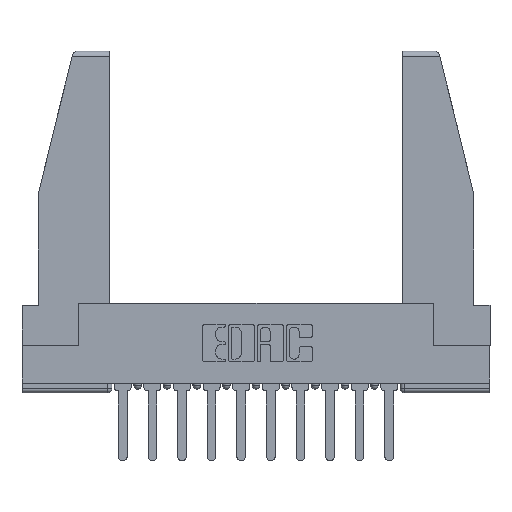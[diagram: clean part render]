
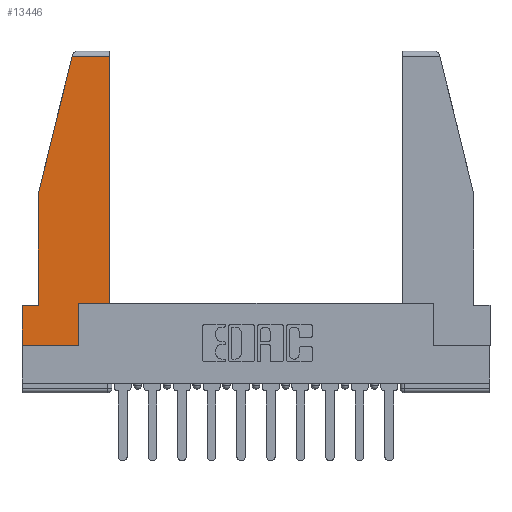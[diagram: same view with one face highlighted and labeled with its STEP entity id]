
A CAD part, top view. The second image highlights one B-rep face of the part: STEP entity #13446.
In plain terms, the highlighted planar face has unit normal (0, 0, 1).
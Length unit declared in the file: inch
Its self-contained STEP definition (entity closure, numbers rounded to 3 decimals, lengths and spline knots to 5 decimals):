
#3 = AXIS2_PLACEMENT_3D ( 'NONE', #6323, #5048, #13193 ) ;
#172 = VECTOR ( 'NONE', #13600, 39.37008 ) ;
#475 = CARTESIAN_POINT ( 'NONE',  ( 0.086, 0.21, 0. ) ) ;
#1074 = VERTEX_POINT ( 'NONE', #9072 ) ;
#1445 = EDGE_CURVE ( 'NONE', #6165, #9530, #11631, .T. ) ;
#3361 = LINE ( 'NONE', #7458, #3905 ) ;
#3769 = ORIENTED_EDGE ( 'NONE', *, *, #1445, .T. ) ;
#3905 = VECTOR ( 'NONE', #4158, 39.37008 ) ;
#3922 = ORIENTED_EDGE ( 'NONE', *, *, #5482, .T. ) ;
#4035 = VERTEX_POINT ( 'NONE', #12150 ) ;
#4087 = LINE ( 'NONE', #4543, #6825 ) ;
#4092 = VECTOR ( 'NONE', #11732, 39.37008 ) ;
#4114 = EDGE_CURVE ( 'NONE', #6142, #10404, #13201, .T. ) ;
#4158 = DIRECTION ( 'NONE',  ( 0., -1., 0. ) ) ;
#4191 = VERTEX_POINT ( 'NONE', #13590 ) ;
#4446 = EDGE_CURVE ( 'NONE', #4035, #11230, #10036, .T. ) ;
#4543 = CARTESIAN_POINT ( 'NONE',  ( 0.297, 0.223, 0. ) ) ;
#4575 = CARTESIAN_POINT ( 'NONE',  ( 0., 1.52, 0. ) ) ;
#5048 = DIRECTION ( 'NONE',  ( 0., 0., 1. ) ) ;
#5482 = EDGE_CURVE ( 'NONE', #1074, #4035, #9086, .T. ) ;
#5774 = CARTESIAN_POINT ( 'NONE',  ( 0.2636, 1.52, 0. ) ) ;
#5826 = ORIENTED_EDGE ( 'NONE', *, *, #15077, .T. ) ;
#5844 = DIRECTION ( 'NONE',  ( -1., 0., 0. ) ) ;
#5978 = EDGE_CURVE ( 'NONE', #11230, #6165, #7572, .T. ) ;
#6142 = VERTEX_POINT ( 'NONE', #8155 ) ;
#6165 = VERTEX_POINT ( 'NONE', #11639 ) ;
#6323 = CARTESIAN_POINT ( 'NONE',  ( 0., 0., 0. ) ) ;
#6807 = LINE ( 'NONE', #6969, #7715 ) ;
#6825 = VECTOR ( 'NONE', #15157, 39.37008 ) ;
#6947 = CARTESIAN_POINT ( 'NONE',  ( 0.086, 0.8, 0. ) ) ;
#6969 = CARTESIAN_POINT ( 'NONE',  ( 0., 0.21, 0. ) ) ;
#7458 = CARTESIAN_POINT ( 'NONE',  ( 0., 0.21, 0. ) ) ;
#7572 = LINE ( 'NONE', #11406, #14068 ) ;
#7689 = CARTESIAN_POINT ( 'NONE',  ( 0., 0., 0. ) ) ;
#7715 = VECTOR ( 'NONE', #15218, 39.37008 ) ;
#8110 = EDGE_LOOP ( 'NONE', ( #3922, #12747, #13913, #3769, #10765, #10985, #11314, #11056, #5826 ) ) ;
#8155 = CARTESIAN_POINT ( 'NONE',  ( 0., 0., 0. ) ) ;
#8229 = EDGE_CURVE ( 'NONE', #9530, #13166, #6807, .T. ) ;
#8375 = EDGE_CURVE ( 'NONE', #10404, #4191, #12878, .T. ) ;
#8838 = DIRECTION ( 'NONE',  ( 1., 0., 0. ) ) ;
#9072 = CARTESIAN_POINT ( 'NONE',  ( 0.461, 0.223, 0. ) ) ;
#9086 = LINE ( 'NONE', #12764, #11678 ) ;
#9530 = VERTEX_POINT ( 'NONE', #475 ) ;
#10036 = LINE ( 'NONE', #4575, #12995 ) ;
#10243 = DIRECTION ( 'NONE',  ( 0., 1., 0. ) ) ;
#10384 = FACE_OUTER_BOUND ( 'NONE', #8110, .T. ) ;
#10404 = VERTEX_POINT ( 'NONE', #14781 ) ;
#10765 = ORIENTED_EDGE ( 'NONE', *, *, #8229, .T. ) ;
#10985 = ORIENTED_EDGE ( 'NONE', *, *, #14771, .T. ) ;
#11056 = ORIENTED_EDGE ( 'NONE', *, *, #8375, .T. ) ;
#11230 = VERTEX_POINT ( 'NONE', #5774 ) ;
#11314 = ORIENTED_EDGE ( 'NONE', *, *, #4114, .T. ) ;
#11406 = CARTESIAN_POINT ( 'NONE',  ( 0.271, 1.55, 0. ) ) ;
#11545 = VECTOR ( 'NONE', #8838, 39.37008 ) ;
#11631 = LINE ( 'NONE', #6947, #4092 ) ;
#11639 = CARTESIAN_POINT ( 'NONE',  ( 0.086, 0.8, 0. ) ) ;
#11678 = VECTOR ( 'NONE', #10243, 39.37008 ) ;
#11732 = DIRECTION ( 'NONE',  ( 0., -1., 0. ) ) ;
#12103 = PLANE ( 'NONE',  #3 ) ;
#12150 = CARTESIAN_POINT ( 'NONE',  ( 0.461, 1.52, 0. ) ) ;
#12481 = DIRECTION ( 'NONE',  ( -0.239, -0.971, 0. ) ) ;
#12747 = ORIENTED_EDGE ( 'NONE', *, *, #4446, .T. ) ;
#12764 = CARTESIAN_POINT ( 'NONE',  ( 0.461, 0.223, 0. ) ) ;
#12878 = LINE ( 'NONE', #14735, #172 ) ;
#12995 = VECTOR ( 'NONE', #5844, 39.37008 ) ;
#13166 = VERTEX_POINT ( 'NONE', #14087 ) ;
#13193 = DIRECTION ( 'NONE',  ( 1., 0., 0. ) ) ;
#13201 = LINE ( 'NONE', #7689, #11545 ) ;
#13446 = ADVANCED_FACE ( 'NONE', ( #10384 ), #12103, .T. ) ;
#13590 = CARTESIAN_POINT ( 'NONE',  ( 0.297, 0.223, 0. ) ) ;
#13600 = DIRECTION ( 'NONE',  ( 0., 1., 0. ) ) ;
#13913 = ORIENTED_EDGE ( 'NONE', *, *, #5978, .T. ) ;
#14068 = VECTOR ( 'NONE', #12481, 39.37008 ) ;
#14087 = CARTESIAN_POINT ( 'NONE',  ( 0., 0.21, 0. ) ) ;
#14735 = CARTESIAN_POINT ( 'NONE',  ( 0.297, 0., 0. ) ) ;
#14771 = EDGE_CURVE ( 'NONE', #13166, #6142, #3361, .T. ) ;
#14781 = CARTESIAN_POINT ( 'NONE',  ( 0.297, 0., 0. ) ) ;
#15077 = EDGE_CURVE ( 'NONE', #4191, #1074, #4087, .T. ) ;
#15157 = DIRECTION ( 'NONE',  ( 1., 0., 0. ) ) ;
#15218 = DIRECTION ( 'NONE',  ( -1., 0., 0. ) ) ;
